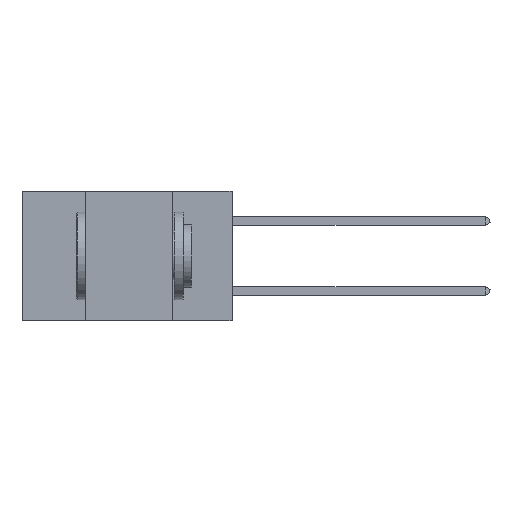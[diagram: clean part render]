
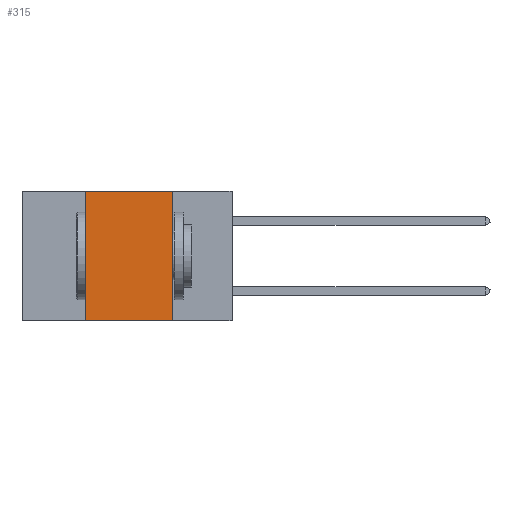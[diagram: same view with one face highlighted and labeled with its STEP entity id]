
A CAD part, left-side view. The second image highlights one B-rep face of the part: STEP entity #315.
In plain terms, the highlighted planar face has unit normal (-1, 0, 0).
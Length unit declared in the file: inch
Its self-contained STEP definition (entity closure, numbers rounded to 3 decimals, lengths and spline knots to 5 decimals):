
#125 = CARTESIAN_POINT ( 'NONE',  ( 0., 0.42, 0. ) ) ;
#315 = ADVANCED_FACE ( 'NONE', ( #2525 ), #4401, .F. ) ;
#785 = LINE ( 'NONE', #1475, #5946 ) ;
#834 = VERTEX_POINT ( 'NONE', #7965 ) ;
#1250 = DIRECTION ( 'NONE',  ( 0., 0., -1. ) ) ;
#1475 = CARTESIAN_POINT ( 'NONE',  ( 0., 0.17, 0. ) ) ;
#1816 = CARTESIAN_POINT ( 'NONE',  ( 0., 0.42, 0. ) ) ;
#1868 = LINE ( 'NONE', #125, #11354 ) ;
#1959 = CARTESIAN_POINT ( 'NONE',  ( 0., 0.6, 0. ) ) ;
#2525 = FACE_OUTER_BOUND ( 'NONE', #7226, .T. ) ;
#2974 = DIRECTION ( 'NONE',  ( 0., -1., 0. ) ) ;
#3111 = DIRECTION ( 'NONE',  ( 0., 0., -1. ) ) ;
#3189 = EDGE_CURVE ( 'NONE', #6174, #8617, #785, .T. ) ;
#3911 = VECTOR ( 'NONE', #6304, 39.37008 ) ;
#4290 = ORIENTED_EDGE ( 'NONE', *, *, #7573, .F. ) ;
#4303 = CARTESIAN_POINT ( 'NONE',  ( 0., 0.6, 0. ) ) ;
#4401 = PLANE ( 'NONE',  #8032 ) ;
#5106 = DIRECTION ( 'NONE',  ( 0., 0., 1. ) ) ;
#5404 = DIRECTION ( 'NONE',  ( 1., 0., 0. ) ) ;
#5523 = VERTEX_POINT ( 'NONE', #1816 ) ;
#5946 = VECTOR ( 'NONE', #1250, 39.37008 ) ;
#6174 = VERTEX_POINT ( 'NONE', #9831 ) ;
#6304 = DIRECTION ( 'NONE',  ( 0., -1., 0. ) ) ;
#6372 = LINE ( 'NONE', #10804, #3911 ) ;
#6447 = VECTOR ( 'NONE', #2974, 39.37008 ) ;
#6453 = ORIENTED_EDGE ( 'NONE', *, *, #3189, .F. ) ;
#7226 = EDGE_LOOP ( 'NONE', ( #6453, #8824, #4290, #11482 ) ) ;
#7275 = EDGE_CURVE ( 'NONE', #5523, #6174, #11235, .T. ) ;
#7573 = EDGE_CURVE ( 'NONE', #834, #5523, #1868, .T. ) ;
#7965 = CARTESIAN_POINT ( 'NONE',  ( 0., 0.42, -0.37 ) ) ;
#8032 = AXIS2_PLACEMENT_3D ( 'NONE', #4303, #5404, #3111 ) ;
#8617 = VERTEX_POINT ( 'NONE', #8644 ) ;
#8644 = CARTESIAN_POINT ( 'NONE',  ( 0., 0.17, -0.37 ) ) ;
#8824 = ORIENTED_EDGE ( 'NONE', *, *, #7275, .F. ) ;
#9831 = CARTESIAN_POINT ( 'NONE',  ( 0., 0.17, 0. ) ) ;
#10804 = CARTESIAN_POINT ( 'NONE',  ( 0., 0.6, -0.37 ) ) ;
#10924 = EDGE_CURVE ( 'NONE', #834, #8617, #6372, .T. ) ;
#11235 = LINE ( 'NONE', #1959, #6447 ) ;
#11354 = VECTOR ( 'NONE', #5106, 39.37008 ) ;
#11482 = ORIENTED_EDGE ( 'NONE', *, *, #10924, .T. ) ;
